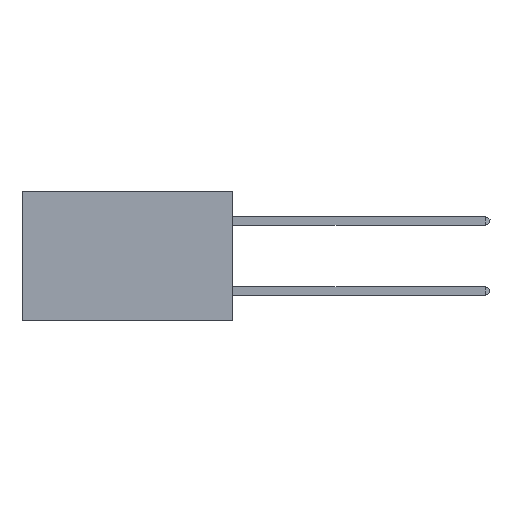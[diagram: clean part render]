
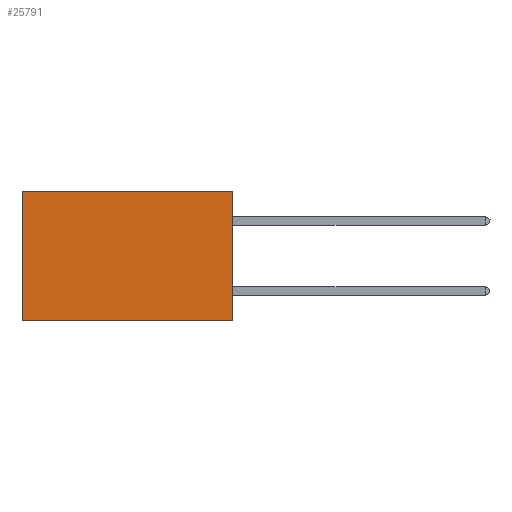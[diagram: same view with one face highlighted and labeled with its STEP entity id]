
A CAD part, left-side view. The second image highlights one B-rep face of the part: STEP entity #25791.
In plain terms, the highlighted planar face has unit normal (-1, 0, 0).
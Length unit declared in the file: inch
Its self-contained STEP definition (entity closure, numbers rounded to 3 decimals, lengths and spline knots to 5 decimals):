
#872 = EDGE_CURVE ( 'NONE', #33642, #27512, #16366, .T. ) ;
#2275 = CARTESIAN_POINT ( 'NONE',  ( 0.2875, 0., 0. ) ) ;
#3877 = CARTESIAN_POINT ( 'NONE',  ( 0.2875, 0.6, 0. ) ) ;
#4098 = CARTESIAN_POINT ( 'NONE',  ( 0.2875, 0., 0. ) ) ;
#4907 = PLANE ( 'NONE',  #9537 ) ;
#5023 = DIRECTION ( 'NONE',  ( 1., 0., 0. ) ) ;
#6065 = CARTESIAN_POINT ( 'NONE',  ( 0.2875, 0.6, -0.37 ) ) ;
#8003 = ORIENTED_EDGE ( 'NONE', *, *, #13843, .F. ) ;
#8290 = LINE ( 'NONE', #34160, #30001 ) ;
#8541 = CARTESIAN_POINT ( 'NONE',  ( 0.2875, 0., -0.37 ) ) ;
#9537 = AXIS2_PLACEMENT_3D ( 'NONE', #34813, #5023, #29268 ) ;
#9960 = VERTEX_POINT ( 'NONE', #6065 ) ;
#10306 = ORIENTED_EDGE ( 'NONE', *, *, #23607, .T. ) ;
#11122 = EDGE_CURVE ( 'NONE', #33642, #32623, #28996, .T. ) ;
#12797 = VECTOR ( 'NONE', #17752, 39.37008 ) ;
#13843 = EDGE_CURVE ( 'NONE', #32623, #9960, #8290, .T. ) ;
#13997 = EDGE_LOOP ( 'NONE', ( #10306, #8003, #22189, #19963 ) ) ;
#15428 = DIRECTION ( 'NONE',  ( 0., 1., 0. ) ) ;
#16366 = LINE ( 'NONE', #22510, #29918 ) ;
#17577 = DIRECTION ( 'NONE',  ( 0., 1., 0. ) ) ;
#17752 = DIRECTION ( 'NONE',  ( 0., 0., -1. ) ) ;
#19963 = ORIENTED_EDGE ( 'NONE', *, *, #872, .T. ) ;
#22189 = ORIENTED_EDGE ( 'NONE', *, *, #11122, .F. ) ;
#22510 = CARTESIAN_POINT ( 'NONE',  ( 0.2875, 0., 0. ) ) ;
#23607 = EDGE_CURVE ( 'NONE', #27512, #9960, #27784, .T. ) ;
#23984 = VECTOR ( 'NONE', #35054, 39.37008 ) ;
#25791 = ADVANCED_FACE ( 'NONE', ( #27781 ), #4907, .F. ) ;
#27512 = VERTEX_POINT ( 'NONE', #31173 ) ;
#27781 = FACE_OUTER_BOUND ( 'NONE', #13997, .T. ) ;
#27784 = LINE ( 'NONE', #3877, #23984 ) ;
#28996 = LINE ( 'NONE', #4098, #12797 ) ;
#29268 = DIRECTION ( 'NONE',  ( 0., 0., -1. ) ) ;
#29918 = VECTOR ( 'NONE', #17577, 39.37008 ) ;
#30001 = VECTOR ( 'NONE', #15428, 39.37008 ) ;
#31173 = CARTESIAN_POINT ( 'NONE',  ( 0.2875, 0.6, 0. ) ) ;
#32623 = VERTEX_POINT ( 'NONE', #8541 ) ;
#33642 = VERTEX_POINT ( 'NONE', #2275 ) ;
#34160 = CARTESIAN_POINT ( 'NONE',  ( 0.2875, 0., -0.37 ) ) ;
#34813 = CARTESIAN_POINT ( 'NONE',  ( 0.2875, 0., 0. ) ) ;
#35054 = DIRECTION ( 'NONE',  ( 0., 0., -1. ) ) ;
